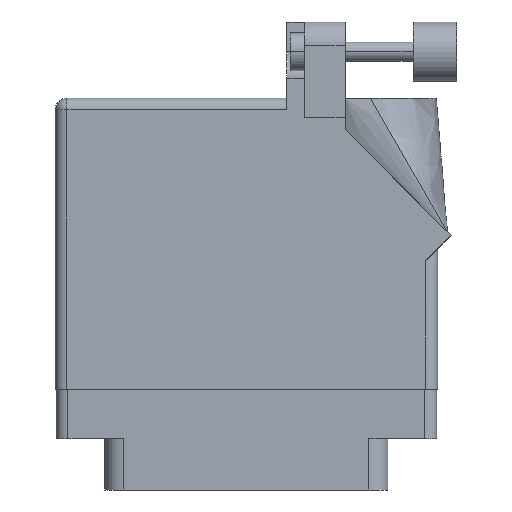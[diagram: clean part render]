
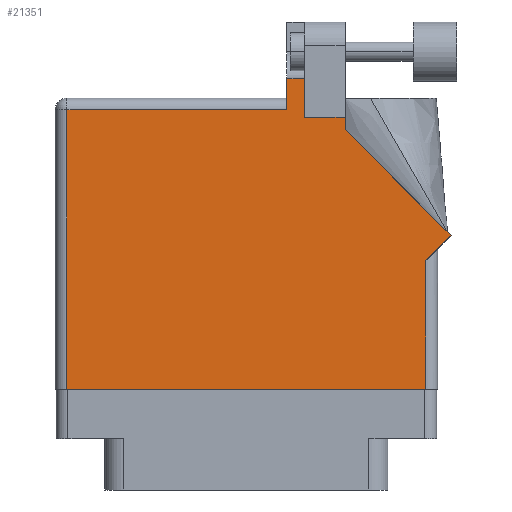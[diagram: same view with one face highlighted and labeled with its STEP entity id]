
A CAD part, front view. The second image highlights one B-rep face of the part: STEP entity #21351.
In plain terms, the highlighted face is planar.
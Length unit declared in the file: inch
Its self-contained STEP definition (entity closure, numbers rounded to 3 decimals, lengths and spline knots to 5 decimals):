
#464 = VECTOR ( 'NONE', #33375, 39.37008 ) ;
#1104 = CARTESIAN_POINT ( 'NONE',  ( 1.217, 1.468, 0. ) ) ;
#1264 = EDGE_CURVE ( 'NONE', #16656, #33126, #32994, .T. ) ;
#1303 = EDGE_CURVE ( 'NONE', #29146, #29706, #16850, .T. ) ;
#1335 = LINE ( 'NONE', #27448, #464 ) ;
#1781 = LINE ( 'NONE', #18396, #9881 ) ;
#2075 = VERTEX_POINT ( 'NONE', #7053 ) ;
#2499 = CARTESIAN_POINT ( 'NONE',  ( 0., 0., 0. ) ) ;
#3606 = ORIENTED_EDGE ( 'NONE', *, *, #28692, .T. ) ;
#4536 = DIRECTION ( 'NONE',  ( 0., -1., 0. ) ) ;
#5396 = CARTESIAN_POINT ( 'NONE',  ( 1.948, 0.737, 0. ) ) ;
#6067 = LINE ( 'NONE', #2499, #31632 ) ;
#7053 = CARTESIAN_POINT ( 'NONE',  ( 1.524, 1.43, 0. ) ) ;
#7196 = LINE ( 'NONE', #13491, #9740 ) ;
#7876 = ORIENTED_EDGE ( 'NONE', *, *, #1264, .T. ) ;
#7887 = ORIENTED_EDGE ( 'NONE', *, *, #10630, .T. ) ;
#8234 = ORIENTED_EDGE ( 'NONE', *, *, #24638, .T. ) ;
#8853 = VERTEX_POINT ( 'NONE', #18287 ) ;
#9616 = DIRECTION ( 'NONE',  ( 0., -1., 0. ) ) ;
#9740 = VECTOR ( 'NONE', #12026, 39.37008 ) ;
#9862 = DIRECTION ( 'NONE',  ( 0., 1., 0. ) ) ;
#9881 = VECTOR ( 'NONE', #26926, 39.37008 ) ;
#9964 = LINE ( 'NONE', #5396, #20193 ) ;
#10448 = ORIENTED_EDGE ( 'NONE', *, *, #29118, .T. ) ;
#10564 = CARTESIAN_POINT ( 'NONE',  ( 0.062, 0., 0. ) ) ;
#10597 = LINE ( 'NONE', #23909, #15309 ) ;
#10630 = EDGE_CURVE ( 'NONE', #2075, #29146, #1335, .T. ) ;
#11001 = PLANE ( 'NONE',  #20257 ) ;
#11828 = EDGE_CURVE ( 'NONE', #33126, #2075, #33625, .T. ) ;
#12026 = DIRECTION ( 'NONE',  ( -1., 0., 0. ) ) ;
#12134 = CARTESIAN_POINT ( 'NONE',  ( 1.311, 1.43, 0. ) ) ;
#13070 = VERTEX_POINT ( 'NONE', #19382 ) ;
#13175 = DIRECTION ( 'NONE',  ( 0., 1., 0. ) ) ;
#13189 = ORIENTED_EDGE ( 'NONE', *, *, #34827, .T. ) ;
#13287 = LINE ( 'NONE', #31439, #26878 ) ;
#13491 = CARTESIAN_POINT ( 'NONE',  ( 0., 1.468, 0. ) ) ;
#14287 = ORIENTED_EDGE ( 'NONE', *, *, #24940, .T. ) ;
#14547 = LINE ( 'NONE', #31501, #23895 ) ;
#15309 = VECTOR ( 'NONE', #4536, 39.37008 ) ;
#16656 = VERTEX_POINT ( 'NONE', #33082 ) ;
#16850 = LINE ( 'NONE', #12134, #18576 ) ;
#17717 = VERTEX_POINT ( 'NONE', #17890 ) ;
#17890 = CARTESIAN_POINT ( 'NONE',  ( 1.948, 0., 0. ) ) ;
#18287 = CARTESIAN_POINT ( 'NONE',  ( 0.062, 1.468, 0. ) ) ;
#18298 = EDGE_LOOP ( 'NONE', ( #32547, #10448, #13189, #8234, #14287, #3606, #28472, #29536, #7876, #22210, #7887 ) ) ;
#18396 = CARTESIAN_POINT ( 'NONE',  ( 1.64177, 1.6315, 0. ) ) ;
#18576 = VECTOR ( 'NONE', #30814, 39.37008 ) ;
#19335 = CARTESIAN_POINT ( 'NONE',  ( 0., 1.53, 0. ) ) ;
#19382 = CARTESIAN_POINT ( 'NONE',  ( 1.948, 0.675, 0. ) ) ;
#19772 = CARTESIAN_POINT ( 'NONE',  ( 2.08071, 0.80771, 0. ) ) ;
#20193 = VECTOR ( 'NONE', #13175, 39.37008 ) ;
#20257 = AXIS2_PLACEMENT_3D ( 'NONE', #19335, #25020, #30022 ) ;
#21351 = ADVANCED_FACE ( 'NONE', ( #24006 ), #11001, .F. ) ;
#21554 = DIRECTION ( 'NONE',  ( 1., 0., 0. ) ) ;
#22210 = ORIENTED_EDGE ( 'NONE', *, *, #11828, .T. ) ;
#22375 = VECTOR ( 'NONE', #33750, 39.37008 ) ;
#22884 = DIRECTION ( 'NONE',  ( 0.707, 0.707, 0. ) ) ;
#23246 = EDGE_CURVE ( 'NONE', #13070, #16656, #13287, .T. ) ;
#23895 = VECTOR ( 'NONE', #9616, 39.37008 ) ;
#23909 = CARTESIAN_POINT ( 'NONE',  ( 0.062, 0., 0. ) ) ;
#24006 = FACE_OUTER_BOUND ( 'NONE', #18298, .T. ) ;
#24638 = EDGE_CURVE ( 'NONE', #29695, #8853, #7196, .T. ) ;
#24940 = EDGE_CURVE ( 'NONE', #8853, #34921, #10597, .T. ) ;
#25020 = DIRECTION ( 'NONE',  ( 0., 0., -1. ) ) ;
#25329 = CARTESIAN_POINT ( 'NONE',  ( 1.217, 1.6315, 0. ) ) ;
#26624 = CARTESIAN_POINT ( 'NONE',  ( 1.524, 1.36442, 0. ) ) ;
#26812 = CARTESIAN_POINT ( 'NONE',  ( 1.311, 1.43, 0. ) ) ;
#26878 = VECTOR ( 'NONE', #22884, 39.37008 ) ;
#26926 = DIRECTION ( 'NONE',  ( -1., 0., 0. ) ) ;
#27448 = CARTESIAN_POINT ( 'NONE',  ( 1.524, 1.43, 0. ) ) ;
#28000 = CARTESIAN_POINT ( 'NONE',  ( 1.311, 1.6315, 0. ) ) ;
#28472 = ORIENTED_EDGE ( 'NONE', *, *, #33606, .T. ) ;
#28692 = EDGE_CURVE ( 'NONE', #34921, #17717, #6067, .T. ) ;
#29118 = EDGE_CURVE ( 'NONE', #29706, #30827, #1781, .T. ) ;
#29146 = VERTEX_POINT ( 'NONE', #26812 ) ;
#29536 = ORIENTED_EDGE ( 'NONE', *, *, #23246, .T. ) ;
#29695 = VERTEX_POINT ( 'NONE', #1104 ) ;
#29706 = VERTEX_POINT ( 'NONE', #28000 ) ;
#30022 = DIRECTION ( 'NONE',  ( -1., 0., 0. ) ) ;
#30814 = DIRECTION ( 'NONE',  ( 0., 1., 0. ) ) ;
#30827 = VERTEX_POINT ( 'NONE', #25329 ) ;
#31439 = CARTESIAN_POINT ( 'NONE',  ( 2.01, 0.737, 0. ) ) ;
#31501 = CARTESIAN_POINT ( 'NONE',  ( 1.217, 1.53, 0. ) ) ;
#31632 = VECTOR ( 'NONE', #21554, 39.37008 ) ;
#32547 = ORIENTED_EDGE ( 'NONE', *, *, #1303, .T. ) ;
#32994 = LINE ( 'NONE', #19772, #22375 ) ;
#33082 = CARTESIAN_POINT ( 'NONE',  ( 2.08071, 0.80771, 0. ) ) ;
#33126 = VERTEX_POINT ( 'NONE', #26624 ) ;
#33375 = DIRECTION ( 'NONE',  ( -1., 0., 0. ) ) ;
#33606 = EDGE_CURVE ( 'NONE', #17717, #13070, #9964, .T. ) ;
#33625 = LINE ( 'NONE', #34588, #34092 ) ;
#33750 = DIRECTION ( 'NONE',  ( -0.707, 0.707, 0. ) ) ;
#34092 = VECTOR ( 'NONE', #9862, 39.37008 ) ;
#34588 = CARTESIAN_POINT ( 'NONE',  ( 1.524, 1.36442, 0. ) ) ;
#34827 = EDGE_CURVE ( 'NONE', #30827, #29695, #14547, .T. ) ;
#34921 = VERTEX_POINT ( 'NONE', #10564 ) ;
